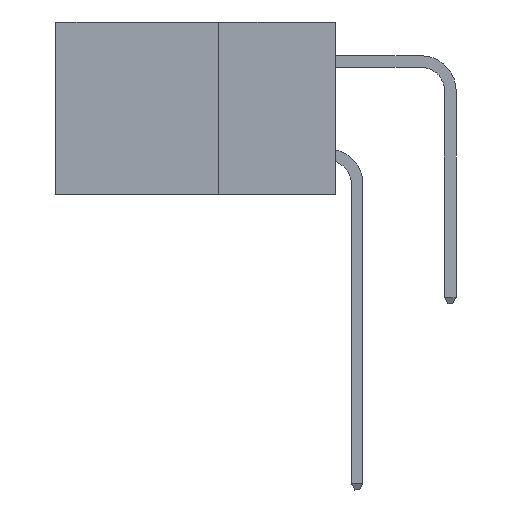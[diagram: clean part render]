
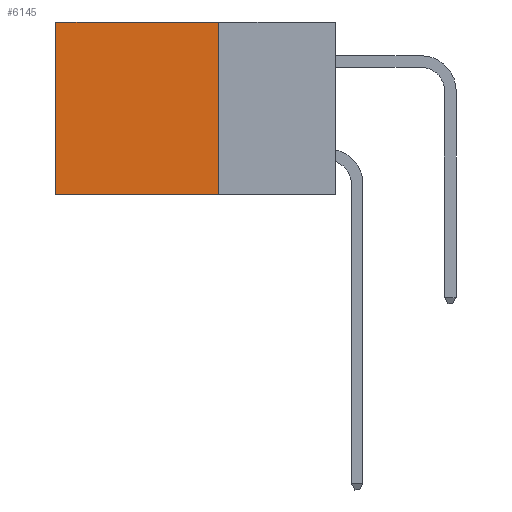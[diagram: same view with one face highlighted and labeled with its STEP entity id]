
A CAD part, left-side view. The second image highlights one B-rep face of the part: STEP entity #6145.
In plain terms, the highlighted planar face has unit normal (-1, 0, 0).
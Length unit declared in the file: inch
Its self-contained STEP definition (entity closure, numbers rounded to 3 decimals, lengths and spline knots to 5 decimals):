
#427 = DIRECTION ( 'NONE',  ( 0., 0., -1. ) ) ;
#892 = CARTESIAN_POINT ( 'NONE',  ( 0.2875, 0.25, -0.37 ) ) ;
#1023 = LINE ( 'NONE', #16409, #15242 ) ;
#1598 = ORIENTED_EDGE ( 'NONE', *, *, #15411, .F. ) ;
#1683 = VECTOR ( 'NONE', #427, 39.37008 ) ;
#2213 = CARTESIAN_POINT ( 'NONE',  ( 0.2875, 0.25, 0. ) ) ;
#3877 = ORIENTED_EDGE ( 'NONE', *, *, #11479, .T. ) ;
#4087 = DIRECTION ( 'NONE',  ( 0., 1., 0. ) ) ;
#4798 = VECTOR ( 'NONE', #16422, 39.37008 ) ;
#6145 = ADVANCED_FACE ( 'NONE', ( #8502 ), #23079, .F. ) ;
#7048 = ORIENTED_EDGE ( 'NONE', *, *, #21149, .T. ) ;
#8502 = FACE_OUTER_BOUND ( 'NONE', #17611, .T. ) ;
#8966 = VERTEX_POINT ( 'NONE', #17397 ) ;
#9399 = VERTEX_POINT ( 'NONE', #892 ) ;
#10793 = DIRECTION ( 'NONE',  ( 0., 0., -1. ) ) ;
#11479 = EDGE_CURVE ( 'NONE', #8966, #13453, #12878, .T. ) ;
#12504 = DIRECTION ( 'NONE',  ( 1., 0., 0. ) ) ;
#12639 = ORIENTED_EDGE ( 'NONE', *, *, #15245, .F. ) ;
#12878 = LINE ( 'NONE', #24737, #22589 ) ;
#13195 = CARTESIAN_POINT ( 'NONE',  ( 0.2875, 0.25, 0. ) ) ;
#13314 = LINE ( 'NONE', #18843, #1683 ) ;
#13453 = VERTEX_POINT ( 'NONE', #17283 ) ;
#14368 = AXIS2_PLACEMENT_3D ( 'NONE', #2213, #12504, #10793 ) ;
#15242 = VECTOR ( 'NONE', #4087, 39.37008 ) ;
#15245 = EDGE_CURVE ( 'NONE', #9399, #13453, #1023, .T. ) ;
#15411 = EDGE_CURVE ( 'NONE', #18241, #9399, #13314, .T. ) ;
#16409 = CARTESIAN_POINT ( 'NONE',  ( 0.2875, 0.25, -0.37 ) ) ;
#16422 = DIRECTION ( 'NONE',  ( 0., 1., 0. ) ) ;
#17283 = CARTESIAN_POINT ( 'NONE',  ( 0.2875, 0.6, -0.37 ) ) ;
#17397 = CARTESIAN_POINT ( 'NONE',  ( 0.2875, 0.6, 0. ) ) ;
#17611 = EDGE_LOOP ( 'NONE', ( #3877, #12639, #1598, #7048 ) ) ;
#18241 = VERTEX_POINT ( 'NONE', #13195 ) ;
#18432 = DIRECTION ( 'NONE',  ( 0., 0., -1. ) ) ;
#18843 = CARTESIAN_POINT ( 'NONE',  ( 0.2875, 0.25, 0. ) ) ;
#21149 = EDGE_CURVE ( 'NONE', #18241, #8966, #21938, .T. ) ;
#21938 = LINE ( 'NONE', #24400, #4798 ) ;
#22589 = VECTOR ( 'NONE', #18432, 39.37008 ) ;
#23079 = PLANE ( 'NONE',  #14368 ) ;
#24400 = CARTESIAN_POINT ( 'NONE',  ( 0.2875, 0.25, 0. ) ) ;
#24737 = CARTESIAN_POINT ( 'NONE',  ( 0.2875, 0.6, 0. ) ) ;
